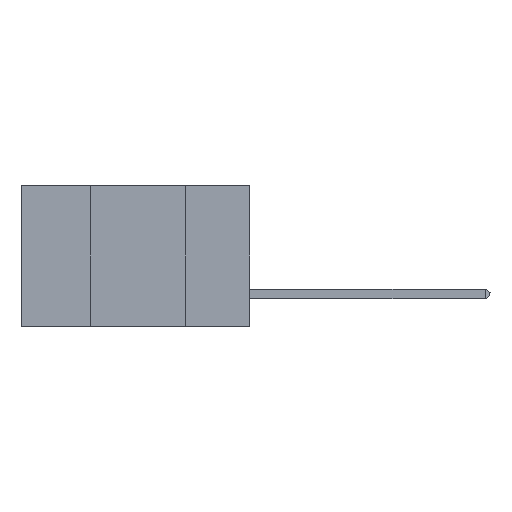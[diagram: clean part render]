
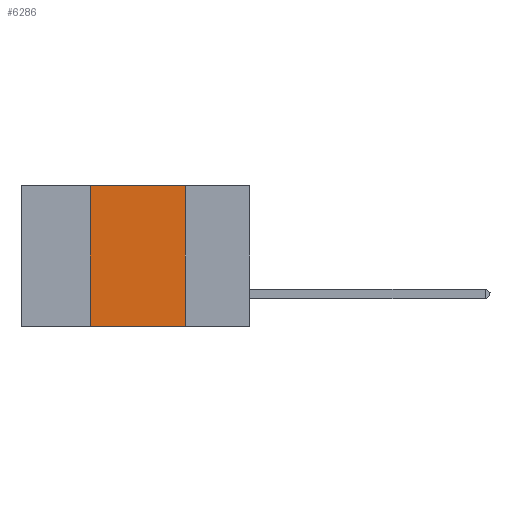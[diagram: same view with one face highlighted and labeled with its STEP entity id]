
A CAD part, left-side view. The second image highlights one B-rep face of the part: STEP entity #6286.
In plain terms, the highlighted planar face has unit normal (-1, 0, 0).
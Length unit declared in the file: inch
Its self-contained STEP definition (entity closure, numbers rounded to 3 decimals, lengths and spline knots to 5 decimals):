
#36 = CARTESIAN_POINT ( 'NONE',  ( 0., 0.17, -0.37 ) ) ;
#1563 = DIRECTION ( 'NONE',  ( 0., 0., 1. ) ) ;
#2750 = FACE_OUTER_BOUND ( 'NONE', #28052, .T. ) ;
#4205 = ORIENTED_EDGE ( 'NONE', *, *, #5093, .T. ) ;
#4615 = LINE ( 'NONE', #7562, #20377 ) ;
#5093 = EDGE_CURVE ( 'NONE', #30755, #30221, #27752, .T. ) ;
#6286 = ADVANCED_FACE ( 'NONE', ( #2750 ), #18234, .F. ) ;
#7238 = CARTESIAN_POINT ( 'NONE',  ( 0., 0.42, 0. ) ) ;
#7562 = CARTESIAN_POINT ( 'NONE',  ( 0., 0.17, 0. ) ) ;
#7589 = CARTESIAN_POINT ( 'NONE',  ( 0., 0.42, -0.37 ) ) ;
#8986 = DIRECTION ( 'NONE',  ( 0., 0., -1. ) ) ;
#11546 = CARTESIAN_POINT ( 'NONE',  ( 0., 0.6, 0. ) ) ;
#13332 = LINE ( 'NONE', #7238, #15070 ) ;
#14598 = VERTEX_POINT ( 'NONE', #30665 ) ;
#15070 = VECTOR ( 'NONE', #1563, 39.37008 ) ;
#15251 = DIRECTION ( 'NONE',  ( 1., 0., 0. ) ) ;
#17731 = DIRECTION ( 'NONE',  ( 0., 0., -1. ) ) ;
#18234 = PLANE ( 'NONE',  #18398 ) ;
#18398 = AXIS2_PLACEMENT_3D ( 'NONE', #34922, #15251, #17731 ) ;
#19175 = CARTESIAN_POINT ( 'NONE',  ( 0., 0.17, 0. ) ) ;
#20199 = CARTESIAN_POINT ( 'NONE',  ( 0., 0.6, -0.37 ) ) ;
#20377 = VECTOR ( 'NONE', #8986, 39.37008 ) ;
#21932 = EDGE_CURVE ( 'NONE', #30755, #14598, #13332, .T. ) ;
#22185 = VECTOR ( 'NONE', #34464, 39.37008 ) ;
#22191 = ORIENTED_EDGE ( 'NONE', *, *, #21932, .F. ) ;
#22200 = EDGE_CURVE ( 'NONE', #14598, #29139, #31891, .T. ) ;
#24216 = VECTOR ( 'NONE', #29206, 39.37008 ) ;
#27752 = LINE ( 'NONE', #20199, #24216 ) ;
#28052 = EDGE_LOOP ( 'NONE', ( #31174, #33236, #22191, #4205 ) ) ;
#29139 = VERTEX_POINT ( 'NONE', #19175 ) ;
#29206 = DIRECTION ( 'NONE',  ( 0., -1., 0. ) ) ;
#30221 = VERTEX_POINT ( 'NONE', #36 ) ;
#30665 = CARTESIAN_POINT ( 'NONE',  ( 0., 0.42, 0. ) ) ;
#30755 = VERTEX_POINT ( 'NONE', #7589 ) ;
#31174 = ORIENTED_EDGE ( 'NONE', *, *, #36005, .F. ) ;
#31891 = LINE ( 'NONE', #11546, #22185 ) ;
#33236 = ORIENTED_EDGE ( 'NONE', *, *, #22200, .F. ) ;
#34464 = DIRECTION ( 'NONE',  ( 0., -1., 0. ) ) ;
#34922 = CARTESIAN_POINT ( 'NONE',  ( 0., 0.6, 0. ) ) ;
#36005 = EDGE_CURVE ( 'NONE', #29139, #30221, #4615, .T. ) ;
